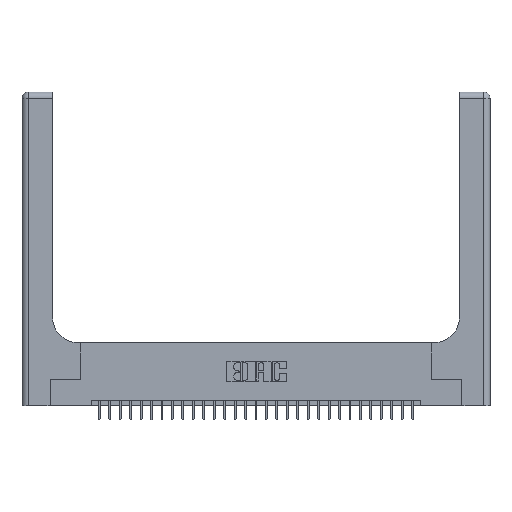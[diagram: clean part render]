
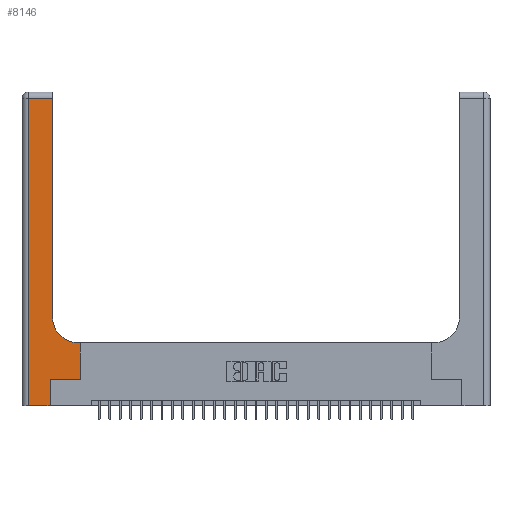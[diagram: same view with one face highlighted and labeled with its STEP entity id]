
A CAD part, top view. The second image highlights one B-rep face of the part: STEP entity #8146.
In plain terms, the highlighted planar face has unit normal (0, 0, 1).
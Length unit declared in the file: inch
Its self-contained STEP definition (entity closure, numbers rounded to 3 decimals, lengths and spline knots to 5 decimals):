
#256 = VECTOR ( 'NONE', #22695, 39.37008 ) ;
#666 = ORIENTED_EDGE ( 'NONE', *, *, #5664, .T. ) ;
#1336 = DIRECTION ( 'NONE',  ( 0., 1., 0. ) ) ;
#1882 = EDGE_CURVE ( 'NONE', #6838, #17394, #11200, .T. ) ;
#1905 = EDGE_CURVE ( 'NONE', #12886, #12918, #8819, .T. ) ;
#2278 = AXIS2_PLACEMENT_3D ( 'NONE', #20137, #8177, #16189 ) ;
#2292 = CARTESIAN_POINT ( 'NONE',  ( 0.5585, 0.6, 0.37 ) ) ;
#2416 = VERTEX_POINT ( 'NONE', #20287 ) ;
#2471 = CARTESIAN_POINT ( 'NONE',  ( 0.269, 0., 0.37 ) ) ;
#2478 = VERTEX_POINT ( 'NONE', #29061 ) ;
#2729 = CARTESIAN_POINT ( 'NONE',  ( 0.06, 3., 0.37 ) ) ;
#2852 = CARTESIAN_POINT ( 'NONE',  ( 0.2915, 0.85, 0.37 ) ) ;
#3196 = DIRECTION ( 'NONE',  ( 0., -1., 0. ) ) ;
#3312 = FACE_OUTER_BOUND ( 'NONE', #23960, .T. ) ;
#3595 = CARTESIAN_POINT ( 'NONE',  ( 0.5585, 0.25, 0.37 ) ) ;
#4032 = CARTESIAN_POINT ( 'NONE',  ( 0.5585, 0.25, 0.37 ) ) ;
#4738 = CARTESIAN_POINT ( 'NONE',  ( 0., 2.94, 0.37 ) ) ;
#5210 = LINE ( 'NONE', #4738, #9345 ) ;
#5664 = EDGE_CURVE ( 'NONE', #2478, #2416, #25068, .T. ) ;
#5732 = ORIENTED_EDGE ( 'NONE', *, *, #1905, .T. ) ;
#6835 = DIRECTION ( 'NONE',  ( 1., 0., 0. ) ) ;
#6838 = VERTEX_POINT ( 'NONE', #2292 ) ;
#8146 = ADVANCED_FACE ( 'NONE', ( #3312 ), #10542, .F. ) ;
#8177 = DIRECTION ( 'NONE',  ( 0., 0., -1. ) ) ;
#8517 = DIRECTION ( 'NONE',  ( -1., 0., 0. ) ) ;
#8819 = LINE ( 'NONE', #18423, #16981 ) ;
#9207 = VECTOR ( 'NONE', #3196, 39.37008 ) ;
#9345 = VECTOR ( 'NONE', #28666, 39.37008 ) ;
#9816 = CARTESIAN_POINT ( 'NONE',  ( 0.5415, 0.6, 0.37 ) ) ;
#10119 = VECTOR ( 'NONE', #21499, 39.37008 ) ;
#10277 = CARTESIAN_POINT ( 'NONE',  ( 0., 0., 0.37 ) ) ;
#10310 = CARTESIAN_POINT ( 'NONE',  ( 0.2915, 3., 0.37 ) ) ;
#10542 = PLANE ( 'NONE',  #2278 ) ;
#10704 = EDGE_CURVE ( 'NONE', #12918, #6838, #25587, .T. ) ;
#10880 = CARTESIAN_POINT ( 'NONE',  ( 0.2915, 0.6, 0.37 ) ) ;
#11200 = LINE ( 'NONE', #10880, #20467 ) ;
#11965 = EDGE_CURVE ( 'NONE', #2416, #12886, #17092, .T. ) ;
#12045 = VERTEX_POINT ( 'NONE', #22844 ) ;
#12386 = AXIS2_PLACEMENT_3D ( 'NONE', #16428, #28391, #6835 ) ;
#12731 = ORIENTED_EDGE ( 'NONE', *, *, #20800, .T. ) ;
#12886 = VERTEX_POINT ( 'NONE', #15564 ) ;
#12918 = VERTEX_POINT ( 'NONE', #3595 ) ;
#13836 = ORIENTED_EDGE ( 'NONE', *, *, #11965, .T. ) ;
#14865 = CIRCLE ( 'NONE', #12386, 0.25 ) ;
#15206 = LINE ( 'NONE', #10310, #15315 ) ;
#15315 = VECTOR ( 'NONE', #1336, 39.37008 ) ;
#15564 = CARTESIAN_POINT ( 'NONE',  ( 0.269, 0.25, 0.37 ) ) ;
#16189 = DIRECTION ( 'NONE',  ( -1., 0., 0. ) ) ;
#16214 = ORIENTED_EDGE ( 'NONE', *, *, #26778, .T. ) ;
#16298 = VERTEX_POINT ( 'NONE', #18600 ) ;
#16428 = CARTESIAN_POINT ( 'NONE',  ( 0.5415, 0.85, 0.37 ) ) ;
#16981 = VECTOR ( 'NONE', #22827, 39.37008 ) ;
#17092 = LINE ( 'NONE', #2471, #10119 ) ;
#17189 = LINE ( 'NONE', #2729, #9207 ) ;
#17394 = VERTEX_POINT ( 'NONE', #9816 ) ;
#18423 = CARTESIAN_POINT ( 'NONE',  ( 0.269, 0.25, 0.37 ) ) ;
#18600 = CARTESIAN_POINT ( 'NONE',  ( 0.06, 2.94, 0.37 ) ) ;
#19318 = EDGE_CURVE ( 'NONE', #12045, #16298, #5210, .T. ) ;
#20137 = CARTESIAN_POINT ( 'NONE',  ( 0., 3., 0.37 ) ) ;
#20287 = CARTESIAN_POINT ( 'NONE',  ( 0.269, 0., 0.37 ) ) ;
#20467 = VECTOR ( 'NONE', #8517, 39.37008 ) ;
#20609 = VECTOR ( 'NONE', #27801, 39.37008 ) ;
#20800 = EDGE_CURVE ( 'NONE', #17394, #25743, #14865, .T. ) ;
#21461 = ORIENTED_EDGE ( 'NONE', *, *, #1882, .T. ) ;
#21499 = DIRECTION ( 'NONE',  ( 0., 1., 0. ) ) ;
#22695 = DIRECTION ( 'NONE',  ( 1., 0., 0. ) ) ;
#22827 = DIRECTION ( 'NONE',  ( 1., 0., 0. ) ) ;
#22844 = CARTESIAN_POINT ( 'NONE',  ( 0.2915, 2.94, 0.37 ) ) ;
#23960 = EDGE_LOOP ( 'NONE', ( #16214, #23977, #26343, #666, #13836, #5732, #27973, #21461, #12731 ) ) ;
#23977 = ORIENTED_EDGE ( 'NONE', *, *, #19318, .T. ) ;
#23988 = EDGE_CURVE ( 'NONE', #16298, #2478, #17189, .T. ) ;
#25068 = LINE ( 'NONE', #10277, #256 ) ;
#25587 = LINE ( 'NONE', #4032, #20609 ) ;
#25743 = VERTEX_POINT ( 'NONE', #2852 ) ;
#26343 = ORIENTED_EDGE ( 'NONE', *, *, #23988, .T. ) ;
#26778 = EDGE_CURVE ( 'NONE', #25743, #12045, #15206, .T. ) ;
#27801 = DIRECTION ( 'NONE',  ( 0., 1., 0. ) ) ;
#27973 = ORIENTED_EDGE ( 'NONE', *, *, #10704, .T. ) ;
#28391 = DIRECTION ( 'NONE',  ( 0., 0., -1. ) ) ;
#28666 = DIRECTION ( 'NONE',  ( -1., 0., 0. ) ) ;
#29061 = CARTESIAN_POINT ( 'NONE',  ( 0.06, 0., 0.37 ) ) ;
